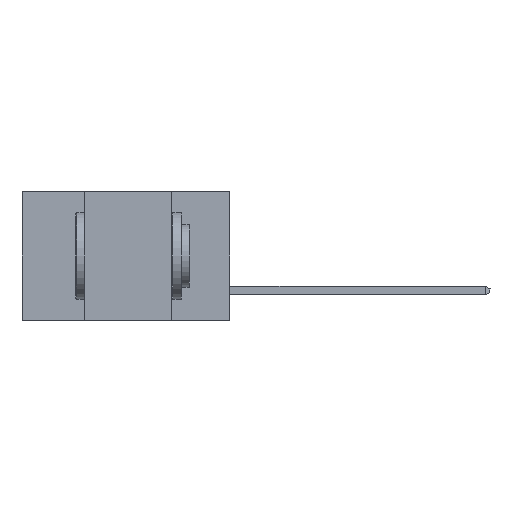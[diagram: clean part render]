
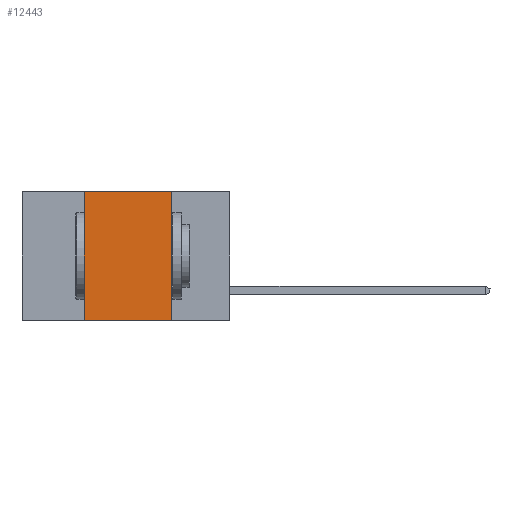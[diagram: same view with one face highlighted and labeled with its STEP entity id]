
A CAD part, left-side view. The second image highlights one B-rep face of the part: STEP entity #12443.
In plain terms, the highlighted planar face has unit normal (-1, 0, 0).
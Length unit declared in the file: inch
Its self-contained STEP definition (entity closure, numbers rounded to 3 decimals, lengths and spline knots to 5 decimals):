
#1229 = LINE ( 'NONE', #5752, #14698 ) ;
#1237 = DIRECTION ( 'NONE',  ( 0., -1., 0. ) ) ;
#1388 = VERTEX_POINT ( 'NONE', #11952 ) ;
#2519 = VERTEX_POINT ( 'NONE', #13189 ) ;
#2572 = AXIS2_PLACEMENT_3D ( 'NONE', #14628, #12538, #9934 ) ;
#2620 = DIRECTION ( 'NONE',  ( 0., -1., 0. ) ) ;
#2822 = ORIENTED_EDGE ( 'NONE', *, *, #13718, .F. ) ;
#3421 = EDGE_CURVE ( 'NONE', #5897, #1388, #1229, .T. ) ;
#3750 = LINE ( 'NONE', #8452, #12344 ) ;
#3865 = VERTEX_POINT ( 'NONE', #4940 ) ;
#4113 = EDGE_LOOP ( 'NONE', ( #2822, #15169, #14000, #9110 ) ) ;
#4133 = FACE_OUTER_BOUND ( 'NONE', #4113, .T. ) ;
#4940 = CARTESIAN_POINT ( 'NONE',  ( 0., 0.17, -0.37 ) ) ;
#5752 = CARTESIAN_POINT ( 'NONE',  ( 0., 0.42, -0.37 ) ) ;
#5897 = VERTEX_POINT ( 'NONE', #6402 ) ;
#6402 = CARTESIAN_POINT ( 'NONE',  ( 0., 0.42, -0.37 ) ) ;
#6720 = VECTOR ( 'NONE', #14859, 39.37008 ) ;
#7066 = CARTESIAN_POINT ( 'NONE',  ( 0., 0.6, -0.37 ) ) ;
#8452 = CARTESIAN_POINT ( 'NONE',  ( 0., 0.6, 0. ) ) ;
#8696 = VECTOR ( 'NONE', #1237, 39.37008 ) ;
#9110 = ORIENTED_EDGE ( 'NONE', *, *, #13761, .T. ) ;
#9934 = DIRECTION ( 'NONE',  ( 0., 0., -1. ) ) ;
#10158 = LINE ( 'NONE', #11403, #6720 ) ;
#10250 = EDGE_CURVE ( 'NONE', #1388, #2519, #3750, .T. ) ;
#10470 = DIRECTION ( 'NONE',  ( 0., 0., 1. ) ) ;
#11403 = CARTESIAN_POINT ( 'NONE',  ( 0., 0.17, -0.37 ) ) ;
#11952 = CARTESIAN_POINT ( 'NONE',  ( 0., 0.42, 0. ) ) ;
#12344 = VECTOR ( 'NONE', #2620, 39.37008 ) ;
#12393 = PLANE ( 'NONE',  #2572 ) ;
#12443 = ADVANCED_FACE ( 'NONE', ( #4133 ), #12393, .F. ) ;
#12538 = DIRECTION ( 'NONE',  ( 1., 0., 0. ) ) ;
#13189 = CARTESIAN_POINT ( 'NONE',  ( 0., 0.17, 0. ) ) ;
#13718 = EDGE_CURVE ( 'NONE', #2519, #3865, #10158, .T. ) ;
#13761 = EDGE_CURVE ( 'NONE', #5897, #3865, #14079, .T. ) ;
#14000 = ORIENTED_EDGE ( 'NONE', *, *, #3421, .F. ) ;
#14079 = LINE ( 'NONE', #7066, #8696 ) ;
#14628 = CARTESIAN_POINT ( 'NONE',  ( 0., 0.6, 0. ) ) ;
#14698 = VECTOR ( 'NONE', #10470, 39.37008 ) ;
#14859 = DIRECTION ( 'NONE',  ( 0., 0., -1. ) ) ;
#15169 = ORIENTED_EDGE ( 'NONE', *, *, #10250, .F. ) ;
